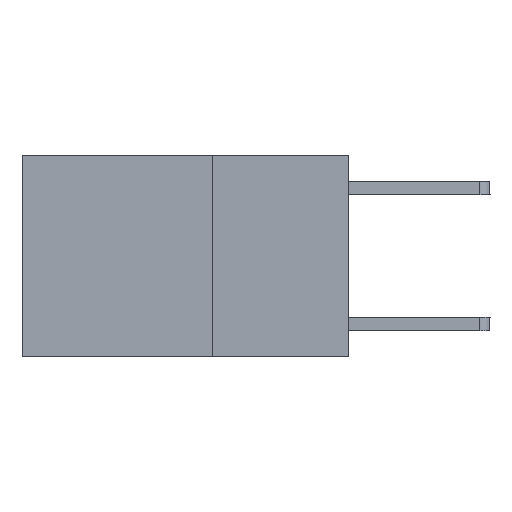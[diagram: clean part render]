
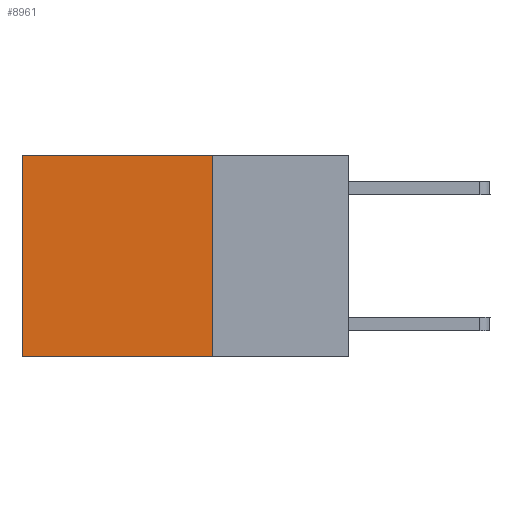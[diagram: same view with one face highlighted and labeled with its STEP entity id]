
A CAD part, left-side view. The second image highlights one B-rep face of the part: STEP entity #8961.
In plain terms, the highlighted planar face has unit normal (-1, 0, 0).
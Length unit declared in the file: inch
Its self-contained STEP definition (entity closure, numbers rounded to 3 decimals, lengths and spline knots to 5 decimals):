
#38 = DIRECTION ( 'NONE',  ( 0., 0., -1. ) ) ;
#451 = ORIENTED_EDGE ( 'NONE', *, *, #6493, .F. ) ;
#799 = ORIENTED_EDGE ( 'NONE', *, *, #8398, .F. ) ;
#826 = VERTEX_POINT ( 'NONE', #7151 ) ;
#1264 = DIRECTION ( 'NONE',  ( 0., 0., -1. ) ) ;
#1300 = DIRECTION ( 'NONE',  ( 0., 1., 0. ) ) ;
#1560 = VECTOR ( 'NONE', #38, 39.37008 ) ;
#1620 = ORIENTED_EDGE ( 'NONE', *, *, #5803, .T. ) ;
#2063 = DIRECTION ( 'NONE',  ( 1., 0., 0. ) ) ;
#3358 = VERTEX_POINT ( 'NONE', #3760 ) ;
#3760 = CARTESIAN_POINT ( 'NONE',  ( 0.2625, 0.6, -0.37 ) ) ;
#4117 = VERTEX_POINT ( 'NONE', #10888 ) ;
#4766 = CARTESIAN_POINT ( 'NONE',  ( 0.2625, 0.25, -0.37 ) ) ;
#4832 = EDGE_LOOP ( 'NONE', ( #1620, #799, #451, #9307 ) ) ;
#5003 = CARTESIAN_POINT ( 'NONE',  ( 0.2625, 0.25, -0.37 ) ) ;
#5803 = EDGE_CURVE ( 'NONE', #4117, #3358, #6917, .T. ) ;
#5807 = PLANE ( 'NONE',  #8281 ) ;
#5818 = VECTOR ( 'NONE', #8824, 39.37008 ) ;
#6493 = EDGE_CURVE ( 'NONE', #826, #8128, #7632, .T. ) ;
#6675 = VECTOR ( 'NONE', #8129, 39.37008 ) ;
#6917 = LINE ( 'NONE', #9995, #6675 ) ;
#7151 = CARTESIAN_POINT ( 'NONE',  ( 0.2625, 0.25, 0. ) ) ;
#7444 = EDGE_CURVE ( 'NONE', #826, #4117, #9670, .T. ) ;
#7632 = LINE ( 'NONE', #8298, #1560 ) ;
#7816 = CARTESIAN_POINT ( 'NONE',  ( 0.2625, 0.25, 0. ) ) ;
#7818 = CARTESIAN_POINT ( 'NONE',  ( 0.2625, 0.25, 0. ) ) ;
#8128 = VERTEX_POINT ( 'NONE', #4766 ) ;
#8129 = DIRECTION ( 'NONE',  ( 0., 0., -1. ) ) ;
#8281 = AXIS2_PLACEMENT_3D ( 'NONE', #7816, #2063, #1264 ) ;
#8298 = CARTESIAN_POINT ( 'NONE',  ( 0.2625, 0.25, 0. ) ) ;
#8398 = EDGE_CURVE ( 'NONE', #8128, #3358, #9592, .T. ) ;
#8824 = DIRECTION ( 'NONE',  ( 0., 1., 0. ) ) ;
#8961 = ADVANCED_FACE ( 'NONE', ( #11297 ), #5807, .F. ) ;
#9307 = ORIENTED_EDGE ( 'NONE', *, *, #7444, .T. ) ;
#9592 = LINE ( 'NONE', #5003, #11611 ) ;
#9670 = LINE ( 'NONE', #7818, #5818 ) ;
#9995 = CARTESIAN_POINT ( 'NONE',  ( 0.2625, 0.6, 0. ) ) ;
#10888 = CARTESIAN_POINT ( 'NONE',  ( 0.2625, 0.6, 0. ) ) ;
#11297 = FACE_OUTER_BOUND ( 'NONE', #4832, .T. ) ;
#11611 = VECTOR ( 'NONE', #1300, 39.37008 ) ;
